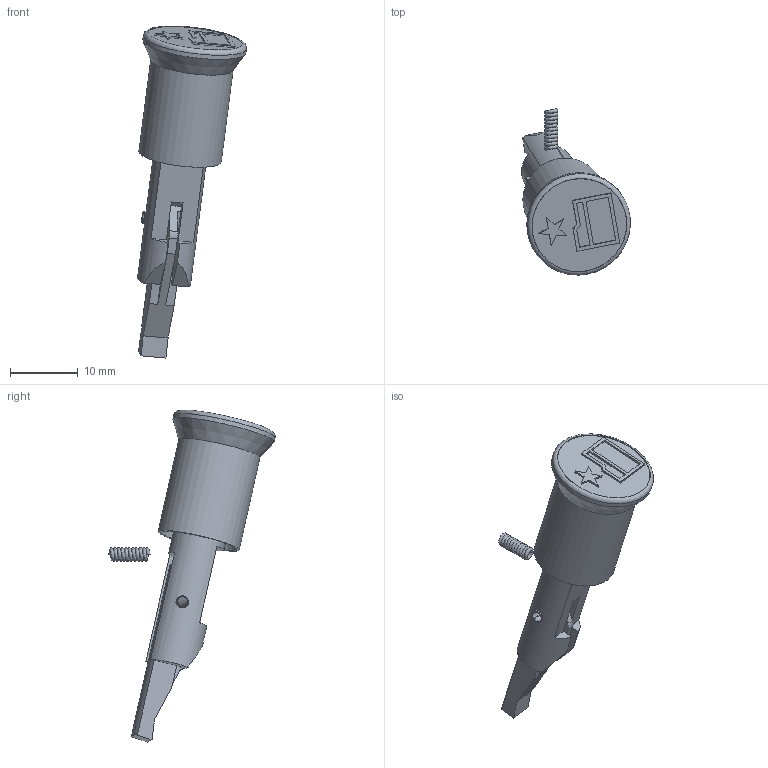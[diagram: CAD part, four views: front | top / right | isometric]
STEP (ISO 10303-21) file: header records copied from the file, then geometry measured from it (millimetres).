
FILE_DESCRIPTION(/* description */ (''),/* implementation_level */ '2;1');
FILE_NAME(/* name */ 'Forward Assist assy.stp',/* time_stamp */ '2018-09-22T00:57:29-05:00',/* author */ ('johne'),/* organization */ (''),/* preprocessor_version */ 'ST-DEVELOPER v16.13',/* originating_system */ 'Autodesk Inventor 2018',/* authorisation */ '');
FILE_SCHEMA (('AUTOMOTIVE_DESIGN { 1 0 10303 214 3 1 1 }'));
Length unit declared in the file: inch
Products named in the file (6): Forward Assist assy; Forward Assist; M16_FORWARD_ASSIST_PAWL_v1; rollpin; pawlpin; pawlspring
Assembly tree (5 placements, depth 2):
  Forward Assist assy
    Forward Assist
    M16_FORWARD_ASSIST_PAWL_v1
    rollpin
    pawlpin
    pawlspring
Bounding box: 16.08 x 24.57 x 49.01 mm (x, y, z)
Volume: 2414 mm3; surface area: 3152.9 mm2
Topology: 5 solids, 5 shells, 92 faces, 229 edges, 154 vertices
Faces by surface type: plane 69, cylinder 14, torus 5, bspline 3, cone 1
Full cylindrical faces by diameter (mm): 1.753 x1, 1.778 x2, 2.032 x1, 2.286 x1, 7.874 x1, 11.506 x1, 12.268 x1, 14.072 x1, 15.342 x1
Entity records: 3974 total; most frequent: CARTESIAN_POINT 1567, DIRECTION 459, ORIENTED_EDGE 424, EDGE_CURVE 212, AXIS2_PLACEMENT_3D 155, LINE 149, VECTOR 149, VERTEX_POINT 149
